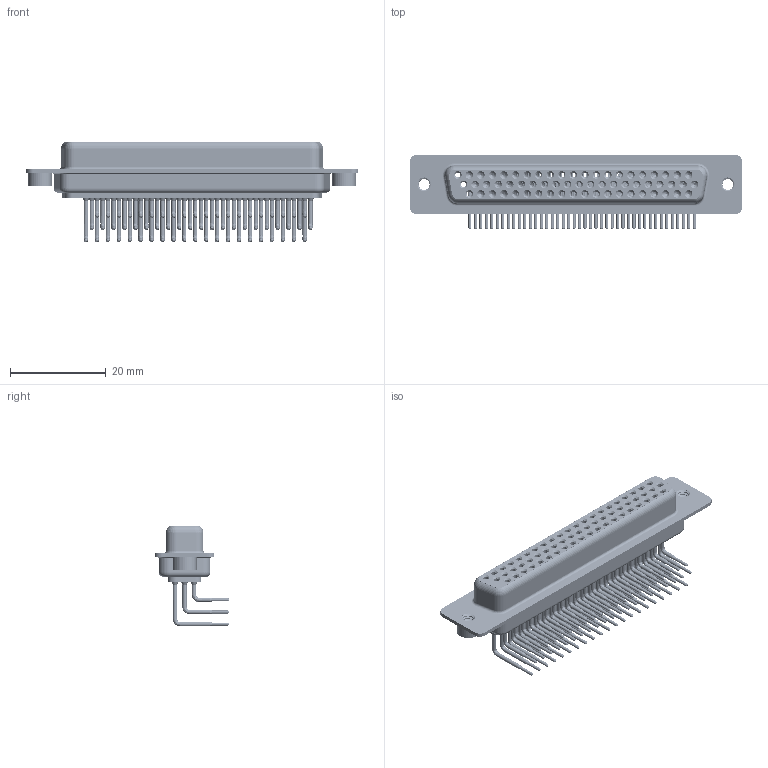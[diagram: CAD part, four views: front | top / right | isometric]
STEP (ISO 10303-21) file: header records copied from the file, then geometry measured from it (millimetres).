
FILE_DESCRIPTION (( 'STEP AP203' ), '1' );
FILE_NAME ('634-M62-663-WN2.STEP', '2018-09-28T04:16:34', ( '' ), ( '' ), 'SwSTEP 2.0', 'SolidWorks 2016', '' );
FILE_SCHEMA (( 'CONFIG_CONTROL_DESIGN' ));
Length unit declared in the file: millimetre
Products named in the file (8): 634M Contact Row 1; 634M Contact Row 2; 634M Contact Row 3; 634M 4-40 Threaded Rivet; 634-M62-663-WN2; 634M Housing_62 Contacts; 634M Shell Front_62 Contacts; 634M Shell Rear_62 Contacts
Assembly tree (67 placements, depth 2):
  634-M62-663-WN2
    634M Housing_62 Contacts
    634M Shell Front_62 Contacts
    634M Shell Rear_62 Contacts
    634M Contact Row 1  x21
    634M Contact Row 2  x21
    634M Contact Row 3  x20
    634M 4-40 Threaded Rivet  x2
Bounding box: 69.4 x 15.6 x 21.02 mm (x, y, z)
Volume: 5405 mm3; surface area: 17867.6 mm2
Topology: 67 solids, 67 shells, 3565 faces, 9057 edges, 5699 vertices
Faces by surface type: cylinder 1563, plane 997, cone 688, bspline 254, torus 63
Entity records: 37999 total; most frequent: CARTESIAN_POINT 7523, DIRECTION 6557, ORIENTED_EDGE 5300, AXIS2_PLACEMENT_3D 2783, EDGE_CURVE 2650, VERTEX_POINT 1693, CIRCLE 1556, EDGE_LOOP 1511
